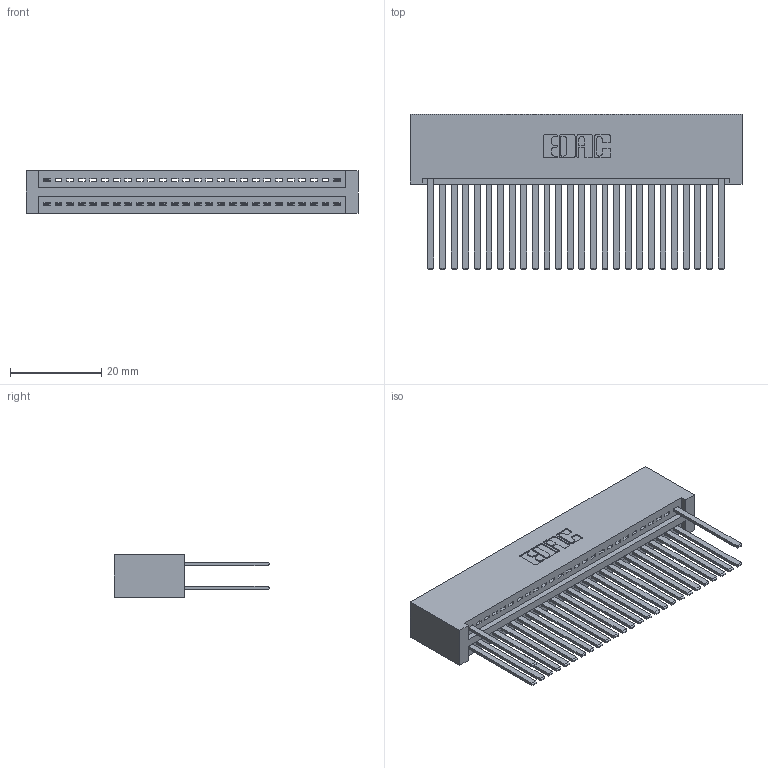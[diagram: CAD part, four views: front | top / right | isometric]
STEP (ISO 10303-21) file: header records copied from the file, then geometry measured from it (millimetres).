
FILE_DESCRIPTION (( 'STEP AP203' ), '1' );
FILE_NAME ('345-052-544-201.STEP', '2018-09-22T23:09:08', ( '' ), ( '' ), 'SwSTEP 2.0', 'SolidWorks 2016', '' );
FILE_SCHEMA (( 'CONFIG_CONTROL_DESIGN' ));
Length unit declared in the file: inch
Products named in the file (3): 345 Part_No Mounting Lugs; 345-292-001_345-293-144; 345-052-544-201
Assembly tree (29 placements, depth 2):
  345-052-544-201
    345 Part_No Mounting Lugs
    345-292-001_345-293-144  x28
Bounding box: 72.64 x 33.96 x 9.4 mm (x, y, z)
Volume: 7700.3 mm3; surface area: 11300.8 mm2
Topology: 29 solids, 29 shells, 1542 faces, 4633 edges, 3050 vertices
Faces by surface type: plane 1056, cylinder 486
Entity records: 21325 total; most frequent: CARTESIAN_POINT 3692, ORIENTED_EDGE 3650, DIRECTION 3241, EDGE_CURVE 1825, VECTOR 1601, LINE 1601, VERTEX_POINT 1214, AXIS2_PLACEMENT_3D 820
